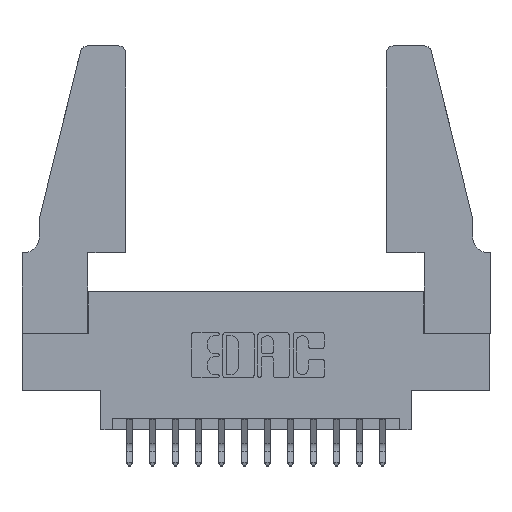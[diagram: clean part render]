
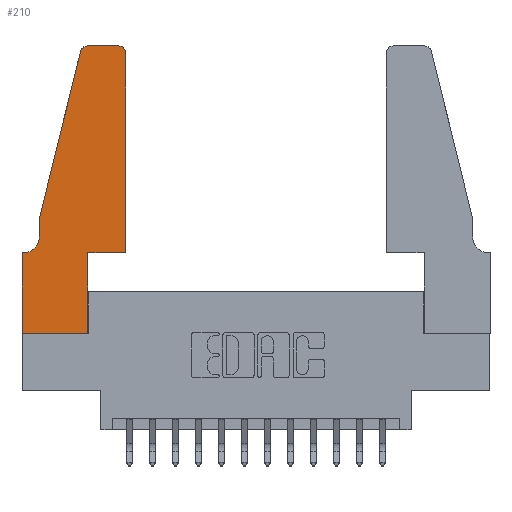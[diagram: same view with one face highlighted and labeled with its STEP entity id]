
A CAD part, top view. The second image highlights one B-rep face of the part: STEP entity #210.
In plain terms, the highlighted planar face has unit normal (0, 0, 1).
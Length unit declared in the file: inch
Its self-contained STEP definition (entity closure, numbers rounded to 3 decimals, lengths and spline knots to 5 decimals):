
#34 = VERTEX_POINT ( 'NONE', #6050 ) ;
#80 = AXIS2_PLACEMENT_3D ( 'NONE', #14426, #7247, #15628 ) ;
#141 = LINE ( 'NONE', #9785, #15775 ) ;
#210 = ADVANCED_FACE ( 'NONE', ( #8668 ), #11035, .T. ) ;
#488 = VERTEX_POINT ( 'NONE', #12909 ) ;
#512 = VERTEX_POINT ( 'NONE', #13639 ) ;
#613 = VERTEX_POINT ( 'NONE', #13097 ) ;
#670 = EDGE_CURVE ( 'NONE', #6640, #1309, #4222, .T. ) ;
#674 = AXIS2_PLACEMENT_3D ( 'NONE', #11312, #4036, #12536 ) ;
#703 = ORIENTED_EDGE ( 'NONE', *, *, #11431, .T. ) ;
#826 = EDGE_CURVE ( 'NONE', #4582, #512, #5602, .T. ) ;
#1222 = LINE ( 'NONE', #3550, #10787 ) ;
#1289 = CARTESIAN_POINT ( 'NONE',  ( 0.0755, 0.42, 0.37 ) ) ;
#1309 = VERTEX_POINT ( 'NONE', #4871 ) ;
#1367 = CARTESIAN_POINT ( 'NONE',  ( 0.2865, 0.35, 0.37 ) ) ;
#1469 = CIRCLE ( 'NONE', #674, 0.03 ) ;
#1607 = LINE ( 'NONE', #6819, #14330 ) ;
#1723 = EDGE_LOOP ( 'NONE', ( #11288, #7742, #703, #9285, #7589, #2395, #12884, #3925, #10814, #12715, #1981, #7675 ) ) ;
#1981 = ORIENTED_EDGE ( 'NONE', *, *, #15617, .T. ) ;
#2284 = DIRECTION ( 'NONE',  ( -1., 0., 0. ) ) ;
#2395 = ORIENTED_EDGE ( 'NONE', *, *, #2991, .T. ) ;
#2481 = EDGE_CURVE ( 'NONE', #3136, #34, #13458, .T. ) ;
#2991 = EDGE_CURVE ( 'NONE', #1309, #9546, #7054, .T. ) ;
#3136 = VERTEX_POINT ( 'NONE', #3910 ) ;
#3550 = CARTESIAN_POINT ( 'NONE',  ( 0., 0., 0.37 ) ) ;
#3614 = EDGE_CURVE ( 'NONE', #13927, #10597, #1222, .T. ) ;
#3754 = VECTOR ( 'NONE', #7774, 39.37008 ) ;
#3910 = CARTESIAN_POINT ( 'NONE',  ( 0.4205, 1.25, 0.37 ) ) ;
#3925 = ORIENTED_EDGE ( 'NONE', *, *, #3614, .T. ) ;
#4036 = DIRECTION ( 'NONE',  ( 0., 0., 1. ) ) ;
#4091 = EDGE_CURVE ( 'NONE', #9546, #13927, #1607, .T. ) ;
#4222 = CIRCLE ( 'NONE', #13141, 0.07 ) ;
#4377 = CARTESIAN_POINT ( 'NONE',  ( 0.4505, 0.35, 0.37 ) ) ;
#4582 = VERTEX_POINT ( 'NONE', #1367 ) ;
#4647 = DIRECTION ( 'NONE',  ( -0.239, -0.971, 0. ) ) ;
#4838 = DIRECTION ( 'NONE',  ( 0., -1., 0. ) ) ;
#4871 = CARTESIAN_POINT ( 'NONE',  ( 0.0055, 0.35, 0.37 ) ) ;
#4968 = DIRECTION ( 'NONE',  ( 0., 1., 0. ) ) ;
#5599 = VECTOR ( 'NONE', #8078, 39.37008 ) ;
#5602 = LINE ( 'NONE', #9377, #14427 ) ;
#5814 = EDGE_CURVE ( 'NONE', #15328, #3136, #7357, .T. ) ;
#6050 = CARTESIAN_POINT ( 'NONE',  ( 0.284, 1.25, 0.37 ) ) ;
#6480 = DIRECTION ( 'NONE',  ( 1., 0., 0. ) ) ;
#6528 = CARTESIAN_POINT ( 'NONE',  ( 0., 0.35, 0.37 ) ) ;
#6640 = VERTEX_POINT ( 'NONE', #1289 ) ;
#6819 = CARTESIAN_POINT ( 'NONE',  ( 0., 0., 0.37 ) ) ;
#6874 = VECTOR ( 'NONE', #4647, 39.37008 ) ;
#7054 = LINE ( 'NONE', #10958, #13073 ) ;
#7247 = DIRECTION ( 'NONE',  ( 0., 0., 1. ) ) ;
#7357 = CIRCLE ( 'NONE', #80, 0.03 ) ;
#7589 = ORIENTED_EDGE ( 'NONE', *, *, #670, .T. ) ;
#7675 = ORIENTED_EDGE ( 'NONE', *, *, #5814, .T. ) ;
#7720 = EDGE_CURVE ( 'NONE', #10597, #4582, #141, .T. ) ;
#7742 = ORIENTED_EDGE ( 'NONE', *, *, #11134, .T. ) ;
#7774 = DIRECTION ( 'NONE',  ( -1., 0., 0. ) ) ;
#7806 = AXIS2_PLACEMENT_3D ( 'NONE', #6528, #10936, #6480 ) ;
#8078 = DIRECTION ( 'NONE',  ( 0., 1., 0. ) ) ;
#8668 = FACE_OUTER_BOUND ( 'NONE', #1723, .T. ) ;
#9137 = EDGE_CURVE ( 'NONE', #488, #6640, #14981, .T. ) ;
#9285 = ORIENTED_EDGE ( 'NONE', *, *, #9137, .T. ) ;
#9377 = CARTESIAN_POINT ( 'NONE',  ( 0.4505, 0.35, 0.37 ) ) ;
#9546 = VERTEX_POINT ( 'NONE', #13969 ) ;
#9576 = DIRECTION ( 'NONE',  ( 1., 0., 0. ) ) ;
#9785 = CARTESIAN_POINT ( 'NONE',  ( 0.2865, 0.35, 0.37 ) ) ;
#10077 = LINE ( 'NONE', #15422, #6874 ) ;
#10329 = CARTESIAN_POINT ( 'NONE',  ( 0.2865, 0., 0.37 ) ) ;
#10597 = VERTEX_POINT ( 'NONE', #10329 ) ;
#10705 = DIRECTION ( 'NONE',  ( 0., 0., -1. ) ) ;
#10706 = CARTESIAN_POINT ( 'NONE',  ( 0., 0., 0.37 ) ) ;
#10787 = VECTOR ( 'NONE', #13302, 39.37008 ) ;
#10814 = ORIENTED_EDGE ( 'NONE', *, *, #7720, .T. ) ;
#10848 = CARTESIAN_POINT ( 'NONE',  ( 0.0755, 0.5, 0.37 ) ) ;
#10936 = DIRECTION ( 'NONE',  ( 0., 0., 1. ) ) ;
#10958 = CARTESIAN_POINT ( 'NONE',  ( 0.0755, 0.35, 0.37 ) ) ;
#11035 = PLANE ( 'NONE',  #7806 ) ;
#11134 = EDGE_CURVE ( 'NONE', #34, #613, #1469, .T. ) ;
#11288 = ORIENTED_EDGE ( 'NONE', *, *, #2481, .T. ) ;
#11312 = CARTESIAN_POINT ( 'NONE',  ( 0.284, 1.22, 0.37 ) ) ;
#11431 = EDGE_CURVE ( 'NONE', #613, #488, #10077, .T. ) ;
#11808 = VECTOR ( 'NONE', #4838, 39.37008 ) ;
#12002 = LINE ( 'NONE', #4377, #5599 ) ;
#12278 = CARTESIAN_POINT ( 'NONE',  ( 0.4505, 1.22, 0.37 ) ) ;
#12536 = DIRECTION ( 'NONE',  ( 1., 0., 0. ) ) ;
#12715 = ORIENTED_EDGE ( 'NONE', *, *, #826, .T. ) ;
#12884 = ORIENTED_EDGE ( 'NONE', *, *, #4091, .T. ) ;
#12909 = CARTESIAN_POINT ( 'NONE',  ( 0.0755, 0.5, 0.37 ) ) ;
#13073 = VECTOR ( 'NONE', #2284, 39.37008 ) ;
#13097 = CARTESIAN_POINT ( 'NONE',  ( 0.25487, 1.22718, 0.37 ) ) ;
#13141 = AXIS2_PLACEMENT_3D ( 'NONE', #13445, #10705, #13415 ) ;
#13302 = DIRECTION ( 'NONE',  ( 1., 0., 0. ) ) ;
#13415 = DIRECTION ( 'NONE',  ( -1., 0., 0. ) ) ;
#13445 = CARTESIAN_POINT ( 'NONE',  ( 0.0055, 0.42, 0.37 ) ) ;
#13458 = LINE ( 'NONE', #14929, #3754 ) ;
#13639 = CARTESIAN_POINT ( 'NONE',  ( 0.4505, 0.35, 0.37 ) ) ;
#13927 = VERTEX_POINT ( 'NONE', #10706 ) ;
#13969 = CARTESIAN_POINT ( 'NONE',  ( 0., 0.35, 0.37 ) ) ;
#14002 = DIRECTION ( 'NONE',  ( 0., -1., 0. ) ) ;
#14330 = VECTOR ( 'NONE', #14002, 39.37008 ) ;
#14426 = CARTESIAN_POINT ( 'NONE',  ( 0.4205, 1.22, 0.37 ) ) ;
#14427 = VECTOR ( 'NONE', #9576, 39.37008 ) ;
#14929 = CARTESIAN_POINT ( 'NONE',  ( 0.2605, 1.25, 0.37 ) ) ;
#14981 = LINE ( 'NONE', #10848, #11808 ) ;
#15328 = VERTEX_POINT ( 'NONE', #12278 ) ;
#15422 = CARTESIAN_POINT ( 'NONE',  ( 0.0755, 0.5, 0.37 ) ) ;
#15617 = EDGE_CURVE ( 'NONE', #512, #15328, #12002, .T. ) ;
#15628 = DIRECTION ( 'NONE',  ( 1., 0., 0. ) ) ;
#15775 = VECTOR ( 'NONE', #4968, 39.37008 ) ;
